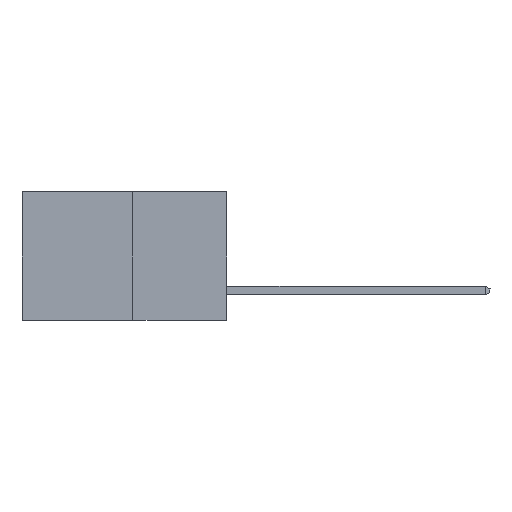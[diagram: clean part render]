
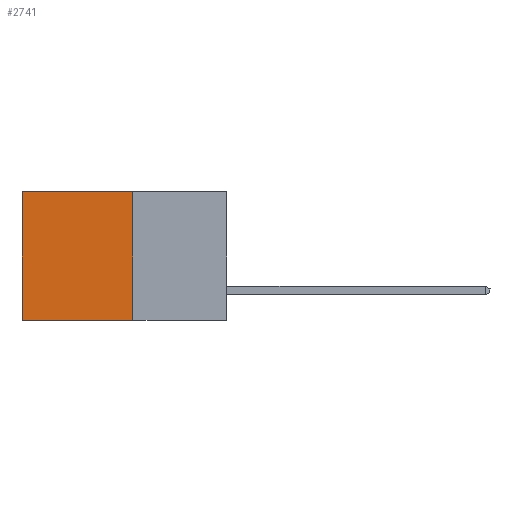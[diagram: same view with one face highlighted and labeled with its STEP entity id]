
A CAD part, left-side view. The second image highlights one B-rep face of the part: STEP entity #2741.
In plain terms, the highlighted planar face has unit normal (-1, 0, 0).
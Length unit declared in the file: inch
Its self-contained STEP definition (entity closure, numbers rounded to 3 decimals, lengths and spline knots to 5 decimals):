
#1881 = DIRECTION ( 'NONE',  ( 0., 1., 0. ) ) ;
#2741 = ADVANCED_FACE ( 'NONE', ( #4998 ), #3411, .F. ) ;
#2793 = DIRECTION ( 'NONE',  ( 1., 0., 0. ) ) ;
#2820 = DIRECTION ( 'NONE',  ( 0., 0., -1. ) ) ;
#2874 = CARTESIAN_POINT ( 'NONE',  ( 0.277, 0.27, -0.37 ) ) ;
#3281 = CARTESIAN_POINT ( 'NONE',  ( 0.277, 0.27, 0. ) ) ;
#3375 = VERTEX_POINT ( 'NONE', #10055 ) ;
#3411 = PLANE ( 'NONE',  #16817 ) ;
#3475 = ORIENTED_EDGE ( 'NONE', *, *, #15934, .F. ) ;
#3807 = LINE ( 'NONE', #3281, #17008 ) ;
#4310 = LINE ( 'NONE', #8121, #14519 ) ;
#4387 = EDGE_CURVE ( 'NONE', #12455, #15279, #16501, .T. ) ;
#4788 = EDGE_LOOP ( 'NONE', ( #5439, #3475, #7138, #15297 ) ) ;
#4998 = FACE_OUTER_BOUND ( 'NONE', #4788, .T. ) ;
#5126 = CARTESIAN_POINT ( 'NONE',  ( 0.277, 0.59, 0. ) ) ;
#5439 = ORIENTED_EDGE ( 'NONE', *, *, #4387, .T. ) ;
#7138 = ORIENTED_EDGE ( 'NONE', *, *, #17041, .F. ) ;
#7509 = DIRECTION ( 'NONE',  ( 0., 0., -1. ) ) ;
#8121 = CARTESIAN_POINT ( 'NONE',  ( 0.277, 0.27, -0.37 ) ) ;
#9614 = VECTOR ( 'NONE', #7509, 39.37008 ) ;
#10055 = CARTESIAN_POINT ( 'NONE',  ( 0.277, 0.27, 0. ) ) ;
#10633 = VERTEX_POINT ( 'NONE', #15577 ) ;
#11267 = VECTOR ( 'NONE', #13764, 39.37008 ) ;
#11436 = CARTESIAN_POINT ( 'NONE',  ( 0.277, 0.59, -0.37 ) ) ;
#12123 = LINE ( 'NONE', #15083, #11267 ) ;
#12455 = VERTEX_POINT ( 'NONE', #5126 ) ;
#13023 = EDGE_CURVE ( 'NONE', #3375, #12455, #3807, .T. ) ;
#13677 = CARTESIAN_POINT ( 'NONE',  ( 0.277, 0.59, -0.37 ) ) ;
#13764 = DIRECTION ( 'NONE',  ( 0., 1., 0. ) ) ;
#14519 = VECTOR ( 'NONE', #17180, 39.37008 ) ;
#15083 = CARTESIAN_POINT ( 'NONE',  ( 0.277, 0.27, -0.37 ) ) ;
#15279 = VERTEX_POINT ( 'NONE', #13677 ) ;
#15297 = ORIENTED_EDGE ( 'NONE', *, *, #13023, .T. ) ;
#15577 = CARTESIAN_POINT ( 'NONE',  ( 0.277, 0.27, -0.37 ) ) ;
#15934 = EDGE_CURVE ( 'NONE', #10633, #15279, #12123, .T. ) ;
#16501 = LINE ( 'NONE', #11436, #9614 ) ;
#16817 = AXIS2_PLACEMENT_3D ( 'NONE', #2874, #2793, #2820 ) ;
#17008 = VECTOR ( 'NONE', #1881, 39.37008 ) ;
#17041 = EDGE_CURVE ( 'NONE', #3375, #10633, #4310, .T. ) ;
#17180 = DIRECTION ( 'NONE',  ( 0., 0., -1. ) ) ;
